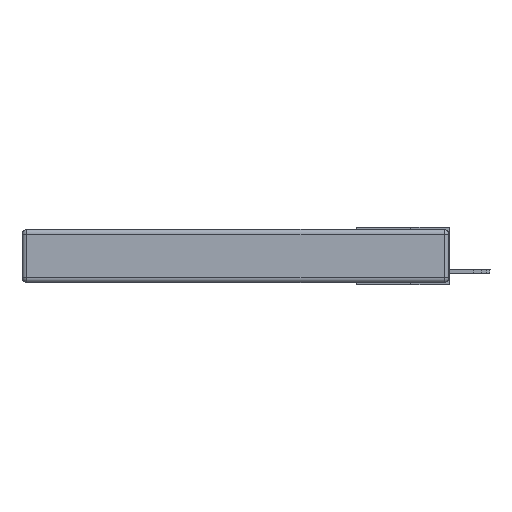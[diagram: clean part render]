
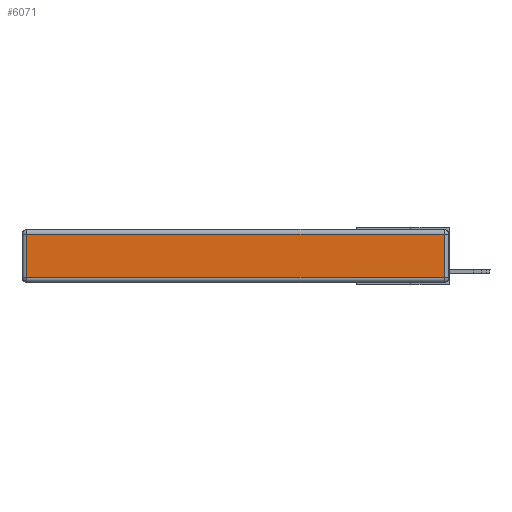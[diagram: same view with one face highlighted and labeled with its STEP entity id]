
A CAD part, left-side view. The second image highlights one B-rep face of the part: STEP entity #6071.
In plain terms, the highlighted planar face has unit normal (-1, 0, 0).
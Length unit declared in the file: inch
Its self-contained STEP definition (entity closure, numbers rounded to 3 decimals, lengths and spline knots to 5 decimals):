
#546 = CARTESIAN_POINT ( 'NONE',  ( 0., 0.03, -0.03 ) ) ;
#853 = DIRECTION ( 'NONE',  ( -1., 0., 0. ) ) ;
#1076 = DIRECTION ( 'NONE',  ( 0., -1., 0. ) ) ;
#1320 = EDGE_CURVE ( 'NONE', #9680, #11036, #7070, .T. ) ;
#1468 = AXIS2_PLACEMENT_3D ( 'NONE', #21606, #853, #13362 ) ;
#2406 = DIRECTION ( 'NONE',  ( 0., 0., -1. ) ) ;
#2986 = ORIENTED_EDGE ( 'NONE', *, *, #12970, .T. ) ;
#4317 = LINE ( 'NONE', #9838, #13150 ) ;
#4923 = LINE ( 'NONE', #16235, #14087 ) ;
#5157 = CARTESIAN_POINT ( 'NONE',  ( 0., 0.03, -0.343 ) ) ;
#5855 = EDGE_CURVE ( 'NONE', #22081, #19645, #4317, .T. ) ;
#6071 = ADVANCED_FACE ( 'NONE', ( #8372 ), #7454, .T. ) ;
#6899 = ORIENTED_EDGE ( 'NONE', *, *, #1320, .T. ) ;
#7070 = LINE ( 'NONE', #18160, #22834 ) ;
#7454 = PLANE ( 'NONE',  #1468 ) ;
#8372 = FACE_OUTER_BOUND ( 'NONE', #15673, .T. ) ;
#8449 = VECTOR ( 'NONE', #19311, 39.37008 ) ;
#9610 = ORIENTED_EDGE ( 'NONE', *, *, #5855, .T. ) ;
#9680 = VERTEX_POINT ( 'NONE', #546 ) ;
#9838 = CARTESIAN_POINT ( 'NONE',  ( 0., 0., -0.313 ) ) ;
#11036 = VERTEX_POINT ( 'NONE', #13634 ) ;
#12970 = EDGE_CURVE ( 'NONE', #19645, #9680, #16222, .T. ) ;
#13150 = VECTOR ( 'NONE', #1076, 39.37008 ) ;
#13362 = DIRECTION ( 'NONE',  ( 0., 0., 1. ) ) ;
#13634 = CARTESIAN_POINT ( 'NONE',  ( 0., 2.72, -0.03 ) ) ;
#14087 = VECTOR ( 'NONE', #2406, 39.37008 ) ;
#14092 = CARTESIAN_POINT ( 'NONE',  ( 0., 0.03, -0.313 ) ) ;
#15014 = CARTESIAN_POINT ( 'NONE',  ( 0., 2.72, -0.313 ) ) ;
#15188 = EDGE_CURVE ( 'NONE', #11036, #22081, #4923, .T. ) ;
#15673 = EDGE_LOOP ( 'NONE', ( #9610, #2986, #6899, #17446 ) ) ;
#16222 = LINE ( 'NONE', #5157, #8449 ) ;
#16235 = CARTESIAN_POINT ( 'NONE',  ( 0., 2.72, -0.343 ) ) ;
#17446 = ORIENTED_EDGE ( 'NONE', *, *, #15188, .T. ) ;
#18160 = CARTESIAN_POINT ( 'NONE',  ( 0., 2.75, -0.03 ) ) ;
#19311 = DIRECTION ( 'NONE',  ( 0., 0., 1. ) ) ;
#19645 = VERTEX_POINT ( 'NONE', #14092 ) ;
#19918 = DIRECTION ( 'NONE',  ( 0., 1., 0. ) ) ;
#21606 = CARTESIAN_POINT ( 'NONE',  ( 0., 0., -0.343 ) ) ;
#22081 = VERTEX_POINT ( 'NONE', #15014 ) ;
#22834 = VECTOR ( 'NONE', #19918, 39.37008 ) ;
